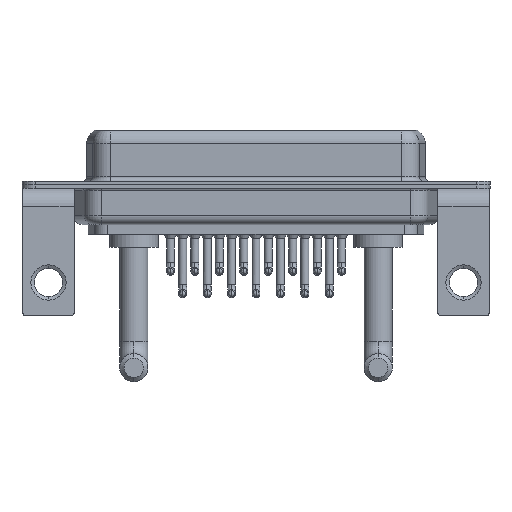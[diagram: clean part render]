
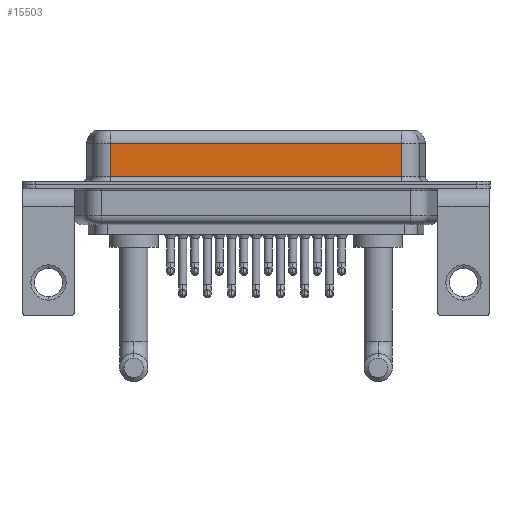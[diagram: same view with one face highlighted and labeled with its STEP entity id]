
A CAD part, front view. The second image highlights one B-rep face of the part: STEP entity #15503.
In plain terms, the highlighted planar face has unit normal (0, -1, 0).
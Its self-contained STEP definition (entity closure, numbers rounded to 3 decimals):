
#479 = DIRECTION ( 'NONE',  ( 1., 0., 0. ) ) ;
#489 = FACE_OUTER_BOUND ( 'NONE', #14677, .T. ) ;
#951 = EDGE_CURVE ( 'NONE', #1768, #13012, #15485, .T. ) ;
#1768 = VERTEX_POINT ( 'NONE', #12033 ) ;
#2112 = ORIENTED_EDGE ( 'NONE', *, *, #12660, .T. ) ;
#2429 = CARTESIAN_POINT ( 'NONE',  ( 40.037, -3.95, 4.65 ) ) ;
#2577 = PLANE ( 'NONE',  #6603 ) ;
#3557 = VERTEX_POINT ( 'NONE', #8206 ) ;
#3980 = ORIENTED_EDGE ( 'NONE', *, *, #951, .T. ) ;
#3982 = CARTESIAN_POINT ( 'NONE',  ( 40.037, -3.95, 0.9 ) ) ;
#4077 = CARTESIAN_POINT ( 'NONE',  ( 40.037, -3.95, 0.9 ) ) ;
#5215 = DIRECTION ( 'NONE',  ( 0., 0., -1. ) ) ;
#5291 = DIRECTION ( 'NONE',  ( 0., 0., -1. ) ) ;
#5478 = VECTOR ( 'NONE', #479, 1000. ) ;
#5750 = DIRECTION ( 'NONE',  ( 0., 0., 1. ) ) ;
#5879 = LINE ( 'NONE', #20624, #9305 ) ;
#6603 = AXIS2_PLACEMENT_3D ( 'NONE', #10551, #9042, #5750 ) ;
#6736 = EDGE_CURVE ( 'NONE', #17863, #13012, #11766, .T. ) ;
#8206 = CARTESIAN_POINT ( 'NONE',  ( 7.013, -3.95, 4.65 ) ) ;
#8574 = CARTESIAN_POINT ( 'NONE',  ( 7.013, -3.95, 6.4 ) ) ;
#9042 = DIRECTION ( 'NONE',  ( 0., 1., 0. ) ) ;
#9305 = VECTOR ( 'NONE', #10550, 1000. ) ;
#10550 = DIRECTION ( 'NONE',  ( -1., 0., 0. ) ) ;
#10551 = CARTESIAN_POINT ( 'NONE',  ( 40.037, -3.95, 6.4 ) ) ;
#11014 = VECTOR ( 'NONE', #5215, 1000. ) ;
#11766 = LINE ( 'NONE', #16577, #11014 ) ;
#12033 = CARTESIAN_POINT ( 'NONE',  ( 7.013, -3.95, 0.9 ) ) ;
#12067 = ORIENTED_EDGE ( 'NONE', *, *, #6736, .F. ) ;
#12660 = EDGE_CURVE ( 'NONE', #17863, #3557, #5879, .T. ) ;
#13012 = VERTEX_POINT ( 'NONE', #4077 ) ;
#14677 = EDGE_LOOP ( 'NONE', ( #12067, #2112, #18814, #3980 ) ) ;
#15342 = VECTOR ( 'NONE', #5291, 1000. ) ;
#15485 = LINE ( 'NONE', #3982, #5478 ) ;
#15503 = ADVANCED_FACE ( 'NONE', ( #489 ), #2577, .F. ) ;
#15759 = EDGE_CURVE ( 'NONE', #3557, #1768, #20051, .T. ) ;
#16577 = CARTESIAN_POINT ( 'NONE',  ( 40.037, -3.95, 6.4 ) ) ;
#17863 = VERTEX_POINT ( 'NONE', #2429 ) ;
#18814 = ORIENTED_EDGE ( 'NONE', *, *, #15759, .T. ) ;
#20051 = LINE ( 'NONE', #8574, #15342 ) ;
#20624 = CARTESIAN_POINT ( 'NONE',  ( 40.037, -3.95, 4.65 ) ) ;
